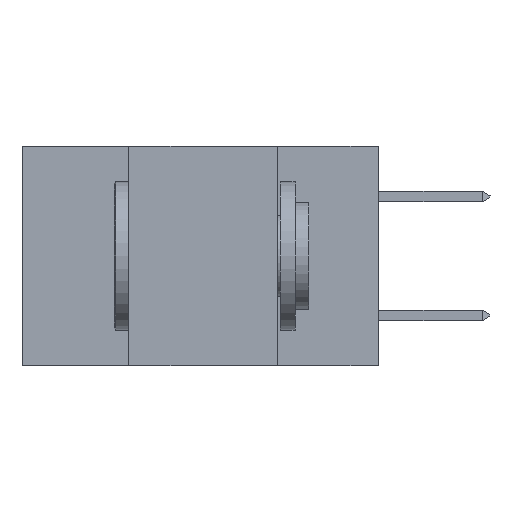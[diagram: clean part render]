
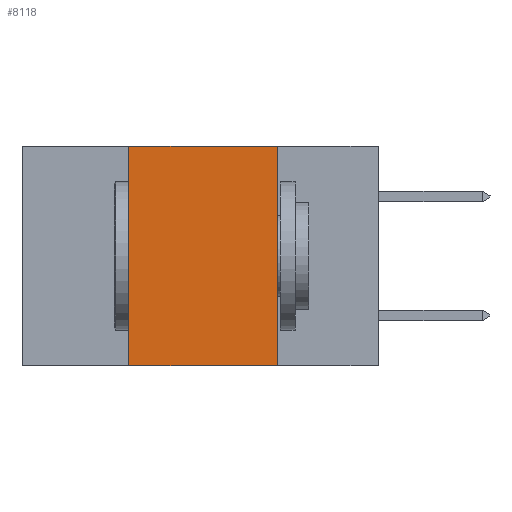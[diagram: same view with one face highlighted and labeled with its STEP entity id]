
A CAD part, left-side view. The second image highlights one B-rep face of the part: STEP entity #8118.
In plain terms, the highlighted planar face has unit normal (-1, 0, 0).
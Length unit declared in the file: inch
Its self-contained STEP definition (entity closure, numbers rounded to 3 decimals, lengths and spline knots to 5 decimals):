
#67 = DIRECTION ( 'NONE',  ( 1., 0., 0. ) ) ;
#171 = EDGE_CURVE ( 'NONE', #2522, #6025, #8838, .T. ) ;
#294 = DIRECTION ( 'NONE',  ( 0., -1., 0. ) ) ;
#795 = PLANE ( 'NONE',  #6571 ) ;
#888 = DIRECTION ( 'NONE',  ( 0., 0., -1. ) ) ;
#2306 = DIRECTION ( 'NONE',  ( 0., 0., -1. ) ) ;
#2461 = CARTESIAN_POINT ( 'NONE',  ( 0., 0.6, -0.37 ) ) ;
#2475 = LINE ( 'NONE', #5698, #9151 ) ;
#2481 = ORIENTED_EDGE ( 'NONE', *, *, #6485, .T. ) ;
#2522 = VERTEX_POINT ( 'NONE', #8527 ) ;
#2684 = ORIENTED_EDGE ( 'NONE', *, *, #171, .F. ) ;
#2695 = EDGE_LOOP ( 'NONE', ( #2684, #4495, #8558, #2481 ) ) ;
#3083 = VECTOR ( 'NONE', #4469, 39.37008 ) ;
#3090 = CARTESIAN_POINT ( 'NONE',  ( 0., 0.42, -0.37 ) ) ;
#3533 = VECTOR ( 'NONE', #294, 39.37008 ) ;
#3840 = VECTOR ( 'NONE', #2306, 39.37008 ) ;
#4469 = DIRECTION ( 'NONE',  ( 0., 0., 1. ) ) ;
#4495 = ORIENTED_EDGE ( 'NONE', *, *, #6166, .F. ) ;
#4507 = FACE_OUTER_BOUND ( 'NONE', #2695, .T. ) ;
#4603 = CARTESIAN_POINT ( 'NONE',  ( 0., 0.42, 0. ) ) ;
#4769 = CARTESIAN_POINT ( 'NONE',  ( 0., 0.42, -0.37 ) ) ;
#5089 = VERTEX_POINT ( 'NONE', #4603 ) ;
#5650 = DIRECTION ( 'NONE',  ( 0., -1., 0. ) ) ;
#5698 = CARTESIAN_POINT ( 'NONE',  ( 0., 0.6, 0. ) ) ;
#6025 = VERTEX_POINT ( 'NONE', #9435 ) ;
#6166 = EDGE_CURVE ( 'NONE', #5089, #2522, #2475, .T. ) ;
#6485 = EDGE_CURVE ( 'NONE', #7292, #6025, #6823, .T. ) ;
#6571 = AXIS2_PLACEMENT_3D ( 'NONE', #6586, #67, #888 ) ;
#6578 = CARTESIAN_POINT ( 'NONE',  ( 0., 0.17, -0.37 ) ) ;
#6586 = CARTESIAN_POINT ( 'NONE',  ( 0., 0.6, 0. ) ) ;
#6823 = LINE ( 'NONE', #2461, #3533 ) ;
#7292 = VERTEX_POINT ( 'NONE', #4769 ) ;
#7650 = EDGE_CURVE ( 'NONE', #7292, #5089, #8096, .T. ) ;
#8096 = LINE ( 'NONE', #3090, #3083 ) ;
#8118 = ADVANCED_FACE ( 'NONE', ( #4507 ), #795, .F. ) ;
#8527 = CARTESIAN_POINT ( 'NONE',  ( 0., 0.17, 0. ) ) ;
#8558 = ORIENTED_EDGE ( 'NONE', *, *, #7650, .F. ) ;
#8838 = LINE ( 'NONE', #6578, #3840 ) ;
#9151 = VECTOR ( 'NONE', #5650, 39.37008 ) ;
#9435 = CARTESIAN_POINT ( 'NONE',  ( 0., 0.17, -0.37 ) ) ;
